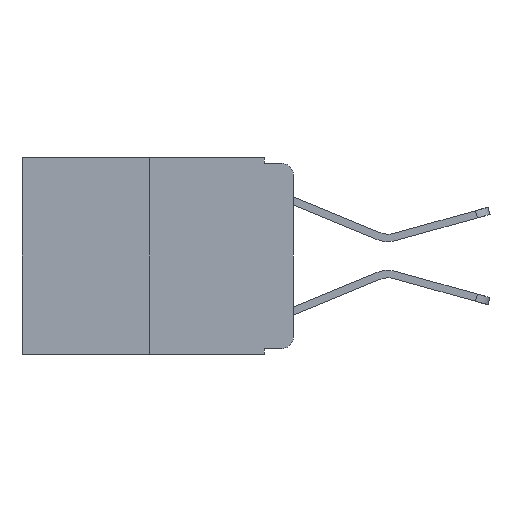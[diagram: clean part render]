
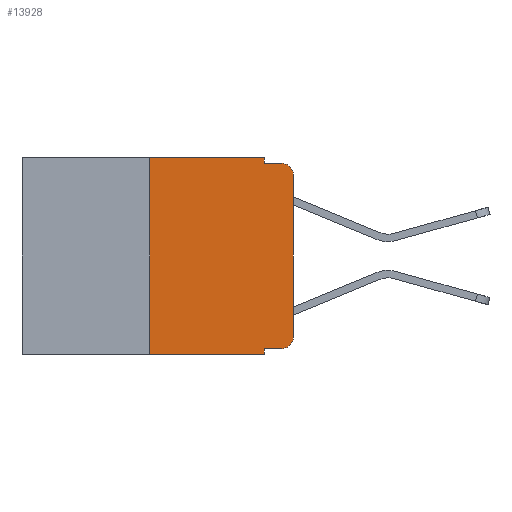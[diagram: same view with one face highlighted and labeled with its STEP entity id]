
A CAD part, left-side view. The second image highlights one B-rep face of the part: STEP entity #13928.
In plain terms, the highlighted planar face has unit normal (-1, 0, 0).
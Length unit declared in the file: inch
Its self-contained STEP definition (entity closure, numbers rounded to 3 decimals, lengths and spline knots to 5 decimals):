
#111 = VECTOR ( 'NONE', #11537, 39.37008 ) ;
#270 = EDGE_CURVE ( 'NONE', #4198, #5239, #9331, .T. ) ;
#460 = DIRECTION ( 'NONE',  ( 0., -1., 0. ) ) ;
#510 = EDGE_CURVE ( 'NONE', #3948, #6801, #9718, .T. ) ;
#675 = EDGE_CURVE ( 'NONE', #10858, #9186, #5441, .T. ) ;
#887 = ORIENTED_EDGE ( 'NONE', *, *, #7831, .T. ) ;
#1038 = EDGE_LOOP ( 'NONE', ( #13131, #3030, #6766, #10356, #7221, #17060, #11124, #4395, #14660, #887 ) ) ;
#1450 = EDGE_CURVE ( 'NONE', #3948, #7166, #13847, .T. ) ;
#1816 = AXIS2_PLACEMENT_3D ( 'NONE', #8046, #6066, #7201 ) ;
#2666 = CIRCLE ( 'NONE', #14858, 0.02 ) ;
#2966 = FACE_OUTER_BOUND ( 'NONE', #1038, .T. ) ;
#3024 = VERTEX_POINT ( 'NONE', #6809 ) ;
#3030 = ORIENTED_EDGE ( 'NONE', *, *, #5813, .T. ) ;
#3856 = CARTESIAN_POINT ( 'NONE',  ( 0., 0.25, 0. ) ) ;
#3864 = VECTOR ( 'NONE', #460, 39.37008 ) ;
#3948 = VERTEX_POINT ( 'NONE', #8091 ) ;
#4198 = VERTEX_POINT ( 'NONE', #14109 ) ;
#4201 = DIRECTION ( 'NONE',  ( 0., -1., 0. ) ) ;
#4395 = ORIENTED_EDGE ( 'NONE', *, *, #11278, .F. ) ;
#4639 = DIRECTION ( 'NONE',  ( 0., 0., -1. ) ) ;
#4876 = EDGE_CURVE ( 'NONE', #5239, #9659, #14462, .T. ) ;
#5239 = VERTEX_POINT ( 'NONE', #9101 ) ;
#5373 = CARTESIAN_POINT ( 'NONE',  ( 0., 0.25, 0. ) ) ;
#5441 = LINE ( 'NONE', #12085, #12012 ) ;
#5813 = EDGE_CURVE ( 'NONE', #3024, #9659, #14974, .T. ) ;
#6066 = DIRECTION ( 'NONE',  ( -1., 0., 0. ) ) ;
#6115 = CARTESIAN_POINT ( 'NONE',  ( 0., 0., 0. ) ) ;
#6706 = PLANE ( 'NONE',  #14125 ) ;
#6766 = ORIENTED_EDGE ( 'NONE', *, *, #4876, .F. ) ;
#6801 = VERTEX_POINT ( 'NONE', #3856 ) ;
#6809 = CARTESIAN_POINT ( 'NONE',  ( 0., 0., -0.03 ) ) ;
#6817 = DIRECTION ( 'NONE',  ( 0., -1., 0. ) ) ;
#7118 = EDGE_CURVE ( 'NONE', #6801, #4198, #13982, .T. ) ;
#7166 = VERTEX_POINT ( 'NONE', #14652 ) ;
#7201 = DIRECTION ( 'NONE',  ( 0., 0., -1. ) ) ;
#7221 = ORIENTED_EDGE ( 'NONE', *, *, #7118, .F. ) ;
#7493 = CARTESIAN_POINT ( 'NONE',  ( 0., 0.02, -0.313 ) ) ;
#7831 = EDGE_CURVE ( 'NONE', #9186, #7896, #2666, .T. ) ;
#7896 = VERTEX_POINT ( 'NONE', #11159 ) ;
#8046 = CARTESIAN_POINT ( 'NONE',  ( 0., 0.02, -0.03 ) ) ;
#8091 = CARTESIAN_POINT ( 'NONE',  ( 0., 0.25, -0.343 ) ) ;
#8131 = DIRECTION ( 'NONE',  ( 1., 0., 0. ) ) ;
#8738 = CARTESIAN_POINT ( 'NONE',  ( 0., 0.051, 0. ) ) ;
#8795 = DIRECTION ( 'NONE',  ( 0., 0., 1. ) ) ;
#8861 = DIRECTION ( 'NONE',  ( 0., 0., -1. ) ) ;
#9101 = CARTESIAN_POINT ( 'NONE',  ( 0., 0.051, -0.01 ) ) ;
#9186 = VERTEX_POINT ( 'NONE', #13184 ) ;
#9331 = LINE ( 'NONE', #11098, #12226 ) ;
#9659 = VERTEX_POINT ( 'NONE', #15172 ) ;
#9674 = LINE ( 'NONE', #6115, #15688 ) ;
#9718 = LINE ( 'NONE', #5373, #12575 ) ;
#10240 = DIRECTION ( 'NONE',  ( 0., 0., 1. ) ) ;
#10356 = ORIENTED_EDGE ( 'NONE', *, *, #270, .F. ) ;
#10825 = VECTOR ( 'NONE', #4201, 39.37008 ) ;
#10858 = VERTEX_POINT ( 'NONE', #13900 ) ;
#11098 = CARTESIAN_POINT ( 'NONE',  ( 0., 0.051, 0. ) ) ;
#11124 = ORIENTED_EDGE ( 'NONE', *, *, #1450, .T. ) ;
#11159 = CARTESIAN_POINT ( 'NONE',  ( 0., 0., -0.313 ) ) ;
#11278 = EDGE_CURVE ( 'NONE', #10858, #7166, #14654, .T. ) ;
#11359 = CARTESIAN_POINT ( 'NONE',  ( 0., 0.473, -0.343 ) ) ;
#11488 = VECTOR ( 'NONE', #4639, 39.37008 ) ;
#11537 = DIRECTION ( 'NONE',  ( 0., -1., 0. ) ) ;
#11549 = CARTESIAN_POINT ( 'NONE',  ( 0., 0.051, -0.01 ) ) ;
#12012 = VECTOR ( 'NONE', #6817, 39.37008 ) ;
#12085 = CARTESIAN_POINT ( 'NONE',  ( 0., 0.051, -0.333 ) ) ;
#12226 = VECTOR ( 'NONE', #15435, 39.37008 ) ;
#12575 = VECTOR ( 'NONE', #8795, 39.37008 ) ;
#13131 = ORIENTED_EDGE ( 'NONE', *, *, #14167, .T. ) ;
#13184 = CARTESIAN_POINT ( 'NONE',  ( 0., 0.02, -0.333 ) ) ;
#13289 = CARTESIAN_POINT ( 'NONE',  ( 0., 0.473, 0. ) ) ;
#13847 = LINE ( 'NONE', #11359, #3864 ) ;
#13900 = CARTESIAN_POINT ( 'NONE',  ( 0., 0.051, -0.333 ) ) ;
#13928 = ADVANCED_FACE ( 'NONE', ( #2966 ), #6706, .F. ) ;
#13982 = LINE ( 'NONE', #13289, #10825 ) ;
#14109 = CARTESIAN_POINT ( 'NONE',  ( 0., 0.051, 0. ) ) ;
#14125 = AXIS2_PLACEMENT_3D ( 'NONE', #15454, #8131, #16652 ) ;
#14167 = EDGE_CURVE ( 'NONE', #7896, #3024, #9674, .T. ) ;
#14462 = LINE ( 'NONE', #11549, #111 ) ;
#14652 = CARTESIAN_POINT ( 'NONE',  ( 0., 0.051, -0.343 ) ) ;
#14654 = LINE ( 'NONE', #8738, #11488 ) ;
#14660 = ORIENTED_EDGE ( 'NONE', *, *, #675, .T. ) ;
#14858 = AXIS2_PLACEMENT_3D ( 'NONE', #7493, #16107, #8861 ) ;
#14974 = CIRCLE ( 'NONE', #1816, 0.02 ) ;
#15172 = CARTESIAN_POINT ( 'NONE',  ( 0., 0.02, -0.01 ) ) ;
#15435 = DIRECTION ( 'NONE',  ( 0., 0., -1. ) ) ;
#15454 = CARTESIAN_POINT ( 'NONE',  ( 0., 0.473, 0. ) ) ;
#15688 = VECTOR ( 'NONE', #10240, 39.37008 ) ;
#16107 = DIRECTION ( 'NONE',  ( -1., 0., 0. ) ) ;
#16652 = DIRECTION ( 'NONE',  ( 0., 0., -1. ) ) ;
#17060 = ORIENTED_EDGE ( 'NONE', *, *, #510, .F. ) ;
